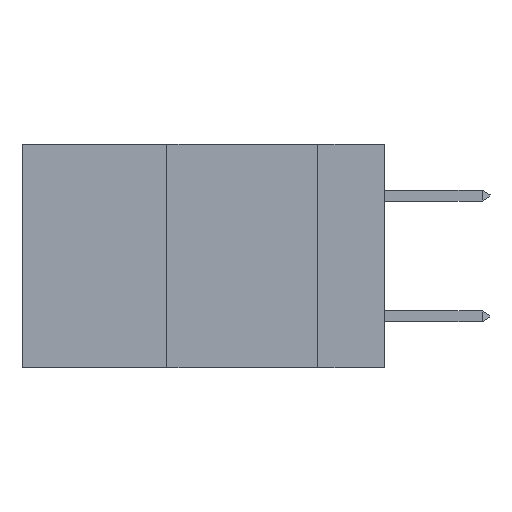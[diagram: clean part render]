
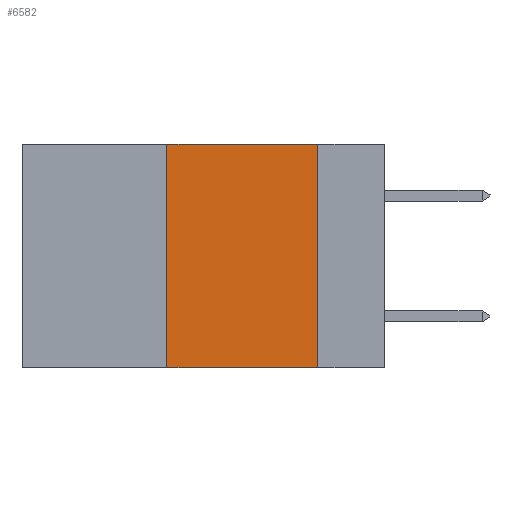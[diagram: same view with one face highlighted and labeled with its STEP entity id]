
A CAD part, left-side view. The second image highlights one B-rep face of the part: STEP entity #6582.
In plain terms, the highlighted planar face has unit normal (-1, 0, 0).
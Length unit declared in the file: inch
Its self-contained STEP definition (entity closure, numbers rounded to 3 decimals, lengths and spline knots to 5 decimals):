
#312 = CARTESIAN_POINT ( 'NONE',  ( 0., 0.6, 0. ) ) ;
#521 = LINE ( 'NONE', #10353, #8315 ) ;
#592 = VECTOR ( 'NONE', #1176, 39.37008 ) ;
#1176 = DIRECTION ( 'NONE',  ( 0., -1., 0. ) ) ;
#1791 = CARTESIAN_POINT ( 'NONE',  ( 0., 0.36, -0.37 ) ) ;
#2323 = VERTEX_POINT ( 'NONE', #1791 ) ;
#2838 = DIRECTION ( 'NONE',  ( 0., 0., 1. ) ) ;
#3470 = AXIS2_PLACEMENT_3D ( 'NONE', #312, #18534, #13072 ) ;
#5250 = FACE_OUTER_BOUND ( 'NONE', #14478, .T. ) ;
#5916 = LINE ( 'NONE', #9066, #8443 ) ;
#6020 = ORIENTED_EDGE ( 'NONE', *, *, #17106, .F. ) ;
#6582 = ADVANCED_FACE ( 'NONE', ( #5250 ), #8470, .F. ) ;
#7600 = VERTEX_POINT ( 'NONE', #14873 ) ;
#7622 = ORIENTED_EDGE ( 'NONE', *, *, #18526, .F. ) ;
#8046 = LINE ( 'NONE', #16076, #17186 ) ;
#8315 = VECTOR ( 'NONE', #10417, 39.37008 ) ;
#8380 = LINE ( 'NONE', #17423, #592 ) ;
#8443 = VECTOR ( 'NONE', #16426, 39.37008 ) ;
#8470 = PLANE ( 'NONE',  #3470 ) ;
#8622 = ORIENTED_EDGE ( 'NONE', *, *, #11670, .F. ) ;
#9066 = CARTESIAN_POINT ( 'NONE',  ( 0., 0.6, -0.37 ) ) ;
#10353 = CARTESIAN_POINT ( 'NONE',  ( 0., 0.11, 0. ) ) ;
#10417 = DIRECTION ( 'NONE',  ( 0., 0., -1. ) ) ;
#10647 = ORIENTED_EDGE ( 'NONE', *, *, #14693, .T. ) ;
#11118 = VERTEX_POINT ( 'NONE', #17498 ) ;
#11670 = EDGE_CURVE ( 'NONE', #2323, #17478, #8046, .T. ) ;
#13072 = DIRECTION ( 'NONE',  ( 0., 0., -1. ) ) ;
#14478 = EDGE_LOOP ( 'NONE', ( #7622, #6020, #8622, #10647 ) ) ;
#14693 = EDGE_CURVE ( 'NONE', #2323, #11118, #5916, .T. ) ;
#14873 = CARTESIAN_POINT ( 'NONE',  ( 0., 0.11, 0. ) ) ;
#15438 = CARTESIAN_POINT ( 'NONE',  ( 0., 0.36, 0. ) ) ;
#16076 = CARTESIAN_POINT ( 'NONE',  ( 0., 0.36, 0. ) ) ;
#16426 = DIRECTION ( 'NONE',  ( 0., -1., 0. ) ) ;
#17106 = EDGE_CURVE ( 'NONE', #17478, #7600, #8380, .T. ) ;
#17186 = VECTOR ( 'NONE', #2838, 39.37008 ) ;
#17423 = CARTESIAN_POINT ( 'NONE',  ( 0., 0.6, 0. ) ) ;
#17478 = VERTEX_POINT ( 'NONE', #15438 ) ;
#17498 = CARTESIAN_POINT ( 'NONE',  ( 0., 0.11, -0.37 ) ) ;
#18526 = EDGE_CURVE ( 'NONE', #7600, #11118, #521, .T. ) ;
#18534 = DIRECTION ( 'NONE',  ( 1., 0., 0. ) ) ;
